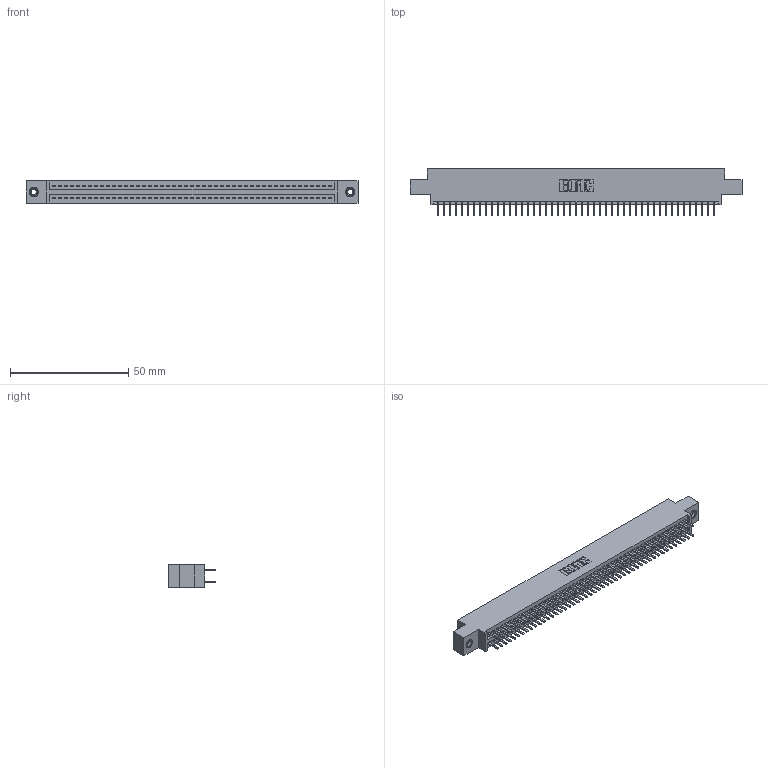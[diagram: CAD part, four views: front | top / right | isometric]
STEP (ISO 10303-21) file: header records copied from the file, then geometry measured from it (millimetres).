
FILE_DESCRIPTION (( 'STEP AP203' ), '1' );
FILE_NAME ('345-094-520-808.STEP', '2018-10-04T23:33:31', ( '' ), ( '' ), 'SwSTEP 2.0', 'SolidWorks 2016', '' );
FILE_SCHEMA (( 'CONFIG_CONTROL_DESIGN' ));
Length unit declared in the file: inch
Products named in the file (4): 345-292-001_345-293-120; 345 Part_0.170 Offset - 0.156 Dia-TI; 345-094-520-808; 345-250-001_345-250-003-102
Assembly tree (97 placements, depth 2):
  345-094-520-808
    345 Part_0.170 Offset - 0.156 Dia-TI
    345-292-001_345-293-120  x94
    345-250-001_345-250-003-102  x2
Bounding box: 140.59 x 19.68 x 9.4 mm (x, y, z)
Volume: 13542.1 mm3; surface area: 20183.4 mm2
Topology: 97 solids, 97 shells, 5266 faces, 15247 edges, 9906 vertices
Faces by surface type: plane 3406, cylinder 1844, cone 12, torus 4
Entity records: 37636 total; most frequent: CARTESIAN_POINT 6299, ORIENTED_EDGE 6214, DIRECTION 5561, EDGE_CURVE 3107, LINE 2763, VECTOR 2763, VERTEX_POINT 2064, AXIS2_PLACEMENT_3D 1399
